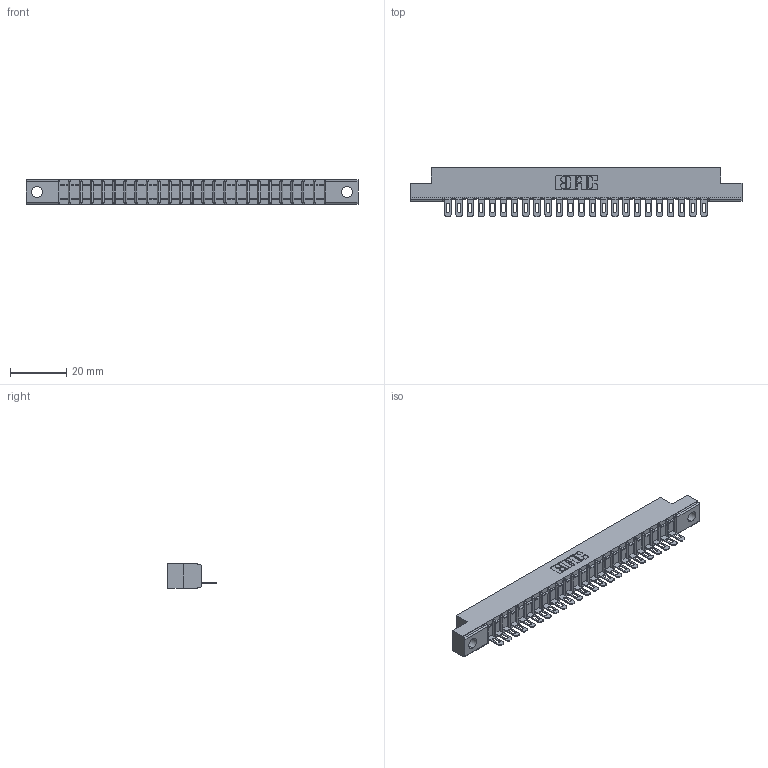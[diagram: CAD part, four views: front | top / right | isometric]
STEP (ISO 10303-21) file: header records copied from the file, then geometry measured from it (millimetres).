
FILE_DESCRIPTION (( 'STEP AP203' ), '1' );
FILE_NAME ('307-024-501-104.STEP', '2018-08-04T06:20:05', ( '' ), ( '' ), 'SwSTEP 2.0', 'SolidWorks 2016', '' );
FILE_SCHEMA (( 'CONFIG_CONTROL_DESIGN' ));
Length unit declared in the file: inch
Products named in the file (3): 307 Part_.156 Dia Mounting Holes; 307-290-002_501; 307-024-501-104
Assembly tree (25 placements, depth 2):
  307-024-501-104
    307 Part_.156 Dia Mounting Holes
    307-290-002_501  x24
Bounding box: 118.11 x 17.42 x 8.71 mm (x, y, z)
Volume: 7713.4 mm3; surface area: 14192.9 mm2
Topology: 25 solids, 25 shells, 1981 faces, 6071 edges, 3978 vertices
Faces by surface type: plane 1140, cylinder 791, sphere 50
Entity records: 24006 total; most frequent: CARTESIAN_POINT 4050, ORIENTED_EDGE 4038, DIRECTION 3939, EDGE_CURVE 2019, VECTOR 1541, LINE 1541, VERTEX_POINT 1310, AXIS2_PLACEMENT_3D 1199
